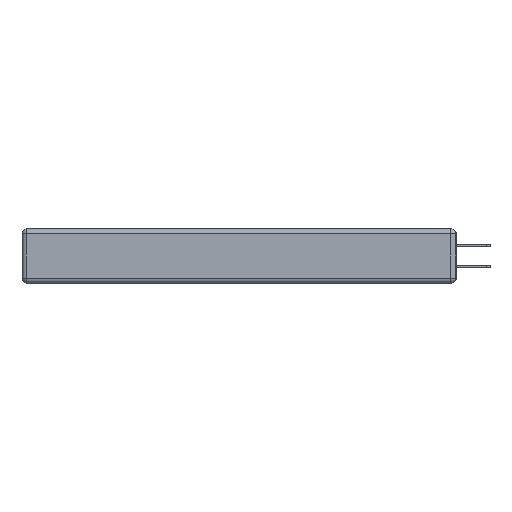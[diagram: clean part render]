
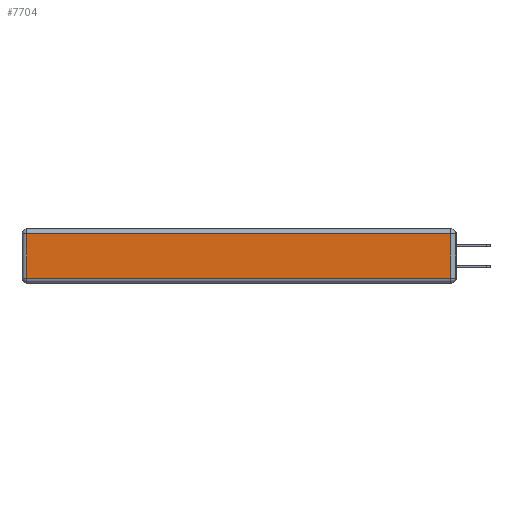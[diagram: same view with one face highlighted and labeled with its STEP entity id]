
A CAD part, left-side view. The second image highlights one B-rep face of the part: STEP entity #7704.
In plain terms, the highlighted planar face has unit normal (-1, 0, 0).
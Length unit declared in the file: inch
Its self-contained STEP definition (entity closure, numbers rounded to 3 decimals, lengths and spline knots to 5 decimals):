
#16 = CARTESIAN_POINT ( 'NONE',  ( 0., 0., -0.313 ) ) ;
#59 = EDGE_LOOP ( 'NONE', ( #3158, #616, #8173, #8793 ) ) ;
#395 = DIRECTION ( 'NONE',  ( 0., 0., 1. ) ) ;
#616 = ORIENTED_EDGE ( 'NONE', *, *, #8044, .T. ) ;
#1599 = VECTOR ( 'NONE', #395, 39.37008 ) ;
#1818 = VERTEX_POINT ( 'NONE', #4111 ) ;
#1862 = CARTESIAN_POINT ( 'NONE',  ( 0., 2.75, -0.03 ) ) ;
#2052 = VECTOR ( 'NONE', #2469, 39.37008 ) ;
#2469 = DIRECTION ( 'NONE',  ( 0., 0., -1. ) ) ;
#3138 = LINE ( 'NONE', #3835, #1599 ) ;
#3158 = ORIENTED_EDGE ( 'NONE', *, *, #10277, .T. ) ;
#3835 = CARTESIAN_POINT ( 'NONE',  ( 0., 0.03, -0.343 ) ) ;
#4111 = CARTESIAN_POINT ( 'NONE',  ( 0., 0.03, -0.313 ) ) ;
#4312 = VECTOR ( 'NONE', #12521, 39.37008 ) ;
#4710 = DIRECTION ( 'NONE',  ( -1., 0., 0. ) ) ;
#4937 = FACE_OUTER_BOUND ( 'NONE', #59, .T. ) ;
#5152 = EDGE_CURVE ( 'NONE', #9337, #7450, #10992, .T. ) ;
#5782 = CARTESIAN_POINT ( 'NONE',  ( 0., 2.72, -0.343 ) ) ;
#7139 = LINE ( 'NONE', #16, #4312 ) ;
#7212 = VECTOR ( 'NONE', #14054, 39.37008 ) ;
#7383 = LINE ( 'NONE', #1862, #7212 ) ;
#7450 = VERTEX_POINT ( 'NONE', #12187 ) ;
#7704 = ADVANCED_FACE ( 'NONE', ( #4937 ), #9392, .T. ) ;
#8044 = EDGE_CURVE ( 'NONE', #1818, #11725, #3138, .T. ) ;
#8173 = ORIENTED_EDGE ( 'NONE', *, *, #13483, .T. ) ;
#8225 = CARTESIAN_POINT ( 'NONE',  ( 0., 0., -0.343 ) ) ;
#8618 = CARTESIAN_POINT ( 'NONE',  ( 0., 2.72, -0.03 ) ) ;
#8793 = ORIENTED_EDGE ( 'NONE', *, *, #5152, .T. ) ;
#9337 = VERTEX_POINT ( 'NONE', #8618 ) ;
#9343 = DIRECTION ( 'NONE',  ( 0., 0., 1. ) ) ;
#9392 = PLANE ( 'NONE',  #10241 ) ;
#10241 = AXIS2_PLACEMENT_3D ( 'NONE', #8225, #4710, #9343 ) ;
#10277 = EDGE_CURVE ( 'NONE', #7450, #1818, #7139, .T. ) ;
#10992 = LINE ( 'NONE', #5782, #2052 ) ;
#11725 = VERTEX_POINT ( 'NONE', #13327 ) ;
#12187 = CARTESIAN_POINT ( 'NONE',  ( 0., 2.72, -0.313 ) ) ;
#12521 = DIRECTION ( 'NONE',  ( 0., -1., 0. ) ) ;
#13327 = CARTESIAN_POINT ( 'NONE',  ( 0., 0.03, -0.03 ) ) ;
#13483 = EDGE_CURVE ( 'NONE', #11725, #9337, #7383, .T. ) ;
#14054 = DIRECTION ( 'NONE',  ( 0., 1., 0. ) ) ;
